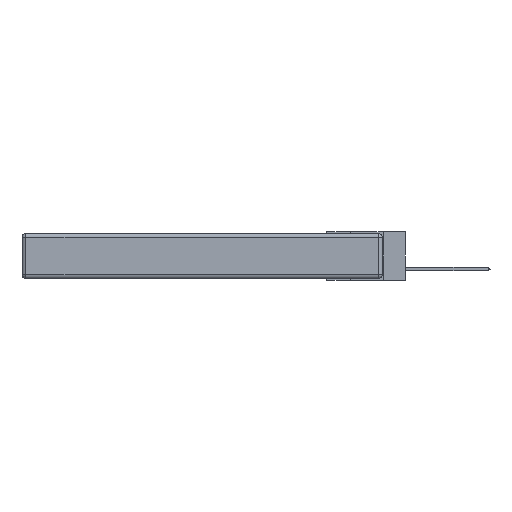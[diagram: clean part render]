
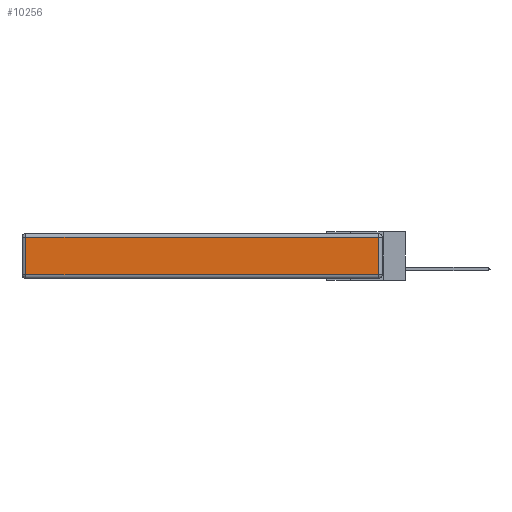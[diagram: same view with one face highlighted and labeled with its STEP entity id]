
A CAD part, left-side view. The second image highlights one B-rep face of the part: STEP entity #10256.
In plain terms, the highlighted planar face has unit normal (-1, 0, 0).
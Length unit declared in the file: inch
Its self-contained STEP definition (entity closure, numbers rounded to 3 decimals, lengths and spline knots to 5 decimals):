
#161 = VECTOR ( 'NONE', #1160, 39.37008 ) ;
#224 = CARTESIAN_POINT ( 'NONE',  ( 0., 0.03, -0.03 ) ) ;
#1160 = DIRECTION ( 'NONE',  ( 0., -1., 0. ) ) ;
#1257 = EDGE_CURVE ( 'NONE', #11780, #8443, #7104, .T. ) ;
#1579 = ORIENTED_EDGE ( 'NONE', *, *, #10061, .T. ) ;
#3067 = DIRECTION ( 'NONE',  ( 0., 0., -1. ) ) ;
#3116 = EDGE_LOOP ( 'NONE', ( #1579, #6103, #12037, #16124 ) ) ;
#3331 = CARTESIAN_POINT ( 'NONE',  ( 0., 0.03, -0.343 ) ) ;
#4083 = CARTESIAN_POINT ( 'NONE',  ( 0., 2.75, -0.03 ) ) ;
#4694 = PLANE ( 'NONE',  #13036 ) ;
#5361 = VECTOR ( 'NONE', #3067, 39.37008 ) ;
#6080 = LINE ( 'NONE', #4083, #12506 ) ;
#6103 = ORIENTED_EDGE ( 'NONE', *, *, #1257, .T. ) ;
#7104 = LINE ( 'NONE', #3331, #7381 ) ;
#7381 = VECTOR ( 'NONE', #14842, 39.37008 ) ;
#7533 = DIRECTION ( 'NONE',  ( 0., 1., 0. ) ) ;
#8443 = VERTEX_POINT ( 'NONE', #224 ) ;
#9074 = CARTESIAN_POINT ( 'NONE',  ( 0., 0.03, -0.313 ) ) ;
#10061 = EDGE_CURVE ( 'NONE', #11143, #11780, #14559, .T. ) ;
#10256 = ADVANCED_FACE ( 'NONE', ( #18346 ), #4694, .T. ) ;
#10999 = CARTESIAN_POINT ( 'NONE',  ( 0., 0., -0.313 ) ) ;
#11143 = VERTEX_POINT ( 'NONE', #17680 ) ;
#11780 = VERTEX_POINT ( 'NONE', #9074 ) ;
#12037 = ORIENTED_EDGE ( 'NONE', *, *, #16877, .T. ) ;
#12506 = VECTOR ( 'NONE', #7533, 39.37008 ) ;
#12564 = LINE ( 'NONE', #16008, #5361 ) ;
#13036 = AXIS2_PLACEMENT_3D ( 'NONE', #19197, #17612, #19265 ) ;
#14559 = LINE ( 'NONE', #10999, #161 ) ;
#14591 = CARTESIAN_POINT ( 'NONE',  ( 0., 2.72, -0.03 ) ) ;
#14842 = DIRECTION ( 'NONE',  ( 0., 0., 1. ) ) ;
#15691 = EDGE_CURVE ( 'NONE', #17224, #11143, #12564, .T. ) ;
#16008 = CARTESIAN_POINT ( 'NONE',  ( 0., 2.72, -0.343 ) ) ;
#16124 = ORIENTED_EDGE ( 'NONE', *, *, #15691, .T. ) ;
#16877 = EDGE_CURVE ( 'NONE', #8443, #17224, #6080, .T. ) ;
#17224 = VERTEX_POINT ( 'NONE', #14591 ) ;
#17612 = DIRECTION ( 'NONE',  ( -1., 0., 0. ) ) ;
#17680 = CARTESIAN_POINT ( 'NONE',  ( 0., 2.72, -0.313 ) ) ;
#18346 = FACE_OUTER_BOUND ( 'NONE', #3116, .T. ) ;
#19197 = CARTESIAN_POINT ( 'NONE',  ( 0., 0., -0.343 ) ) ;
#19265 = DIRECTION ( 'NONE',  ( 0., 0., 1. ) ) ;
